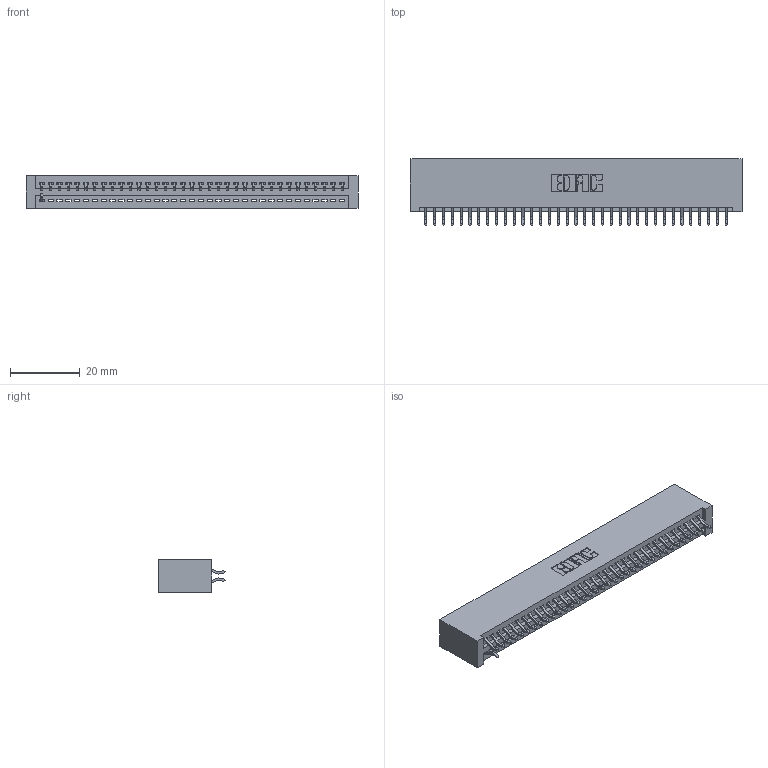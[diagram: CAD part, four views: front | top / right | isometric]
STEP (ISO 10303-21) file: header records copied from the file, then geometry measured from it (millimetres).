
FILE_DESCRIPTION (( 'STEP AP203' ), '1' );
FILE_NAME ('395-070-556-201.STEP', '2018-11-27T00:44:18', ( '' ), ( '' ), 'SwSTEP 2.0', 'SolidWorks 2016', '' );
FILE_SCHEMA (( 'CONFIG_CONTROL_DESIGN' ));
Length unit declared in the file: inch
Products named in the file (3): 395-070-556-201; 345 Part_No Mounting Lugs; 345-292-001_556 Tail
Assembly tree (37 placements, depth 2):
  395-070-556-201
    345 Part_No Mounting Lugs
    345-292-001_556 Tail  x36
Bounding box: 95.5 x 19.24 x 9.4 mm (x, y, z)
Volume: 9520.4 mm3; surface area: 12473.1 mm2
Topology: 37 solids, 37 shells, 2406 faces, 7247 edges, 4782 vertices
Faces by surface type: plane 1646, cylinder 760
Entity records: 27259 total; most frequent: CARTESIAN_POINT 4738, ORIENTED_EDGE 4694, DIRECTION 4131, EDGE_CURVE 2347, VECTOR 2075, LINE 2075, VERTEX_POINT 1562, AXIS2_PLACEMENT_3D 1028
